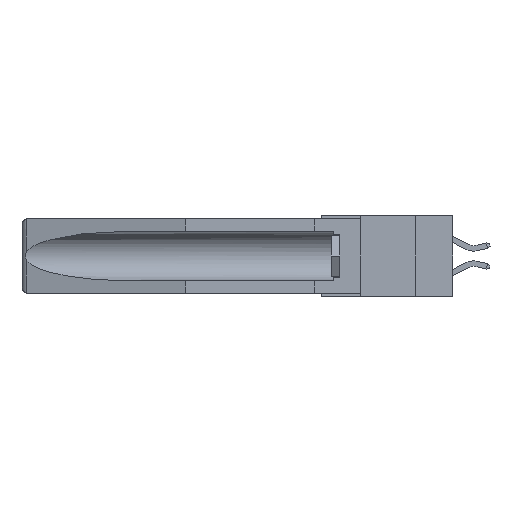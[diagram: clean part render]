
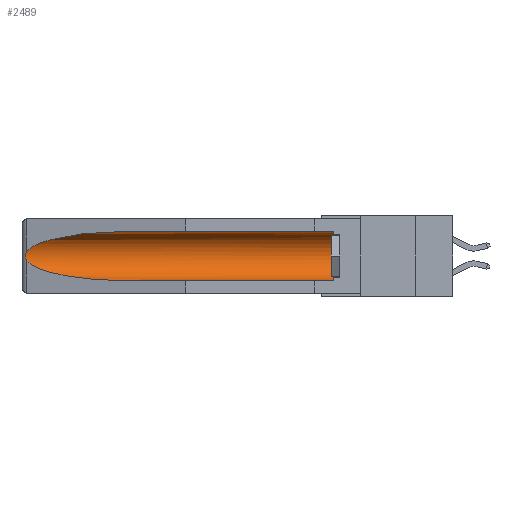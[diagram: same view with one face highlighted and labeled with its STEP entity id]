
A CAD part, left-side view. The second image highlights one B-rep face of the part: STEP entity #2489.
In plain terms, the highlighted cylindrical face has radius 2.857 mm (diameter 5.715 mm), a partial arc.
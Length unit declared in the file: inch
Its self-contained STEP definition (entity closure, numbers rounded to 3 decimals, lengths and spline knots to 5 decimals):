
#273 = VERTEX_POINT ( 'NONE', #5281 ) ;
#656 = EDGE_CURVE ( 'NONE', #273, #11229, #10351, .T. ) ;
#700 = LINE ( 'NONE', #4489, #19668 ) ;
#905 = CARTESIAN_POINT ( 'NONE',  ( 0.26537, 1.52718, -0.19328 ) ) ;
#1743 = EDGE_CURVE ( 'NONE', #6152, #273, #700, .T. ) ;
#2489 = ADVANCED_FACE ( 'NONE', ( #12251 ), #11237, .F. ) ;
#3765 = CARTESIAN_POINT ( 'NONE',  ( 0.26537, 1.52718, -0.19328 ) ) ;
#3939 = EDGE_CURVE ( 'NONE', #9594, #15477, #4488, .T. ) ;
#4488 =( BOUNDED_CURVE ( )  B_SPLINE_CURVE ( 3, ( #6036, #9517, #6104, #21020 ),
 .UNSPECIFIED., .F., .F. ) 
 B_SPLINE_CURVE_WITH_KNOTS ( ( 4, 4 ),
 ( 0.1948, 1.5708 ),
 .UNSPECIFIED. ) 
 CURVE ( )  GEOMETRIC_REPRESENTATION_ITEM ( )  RATIONAL_B_SPLINE_CURVE ( ( 1., 0.848, 0.848, 1. ) ) 
 REPRESENTATION_ITEM ( '' )  );
#4489 = CARTESIAN_POINT ( 'NONE',  ( 0.155, -0.30754, -0.059 ) ) ;
#5281 = CARTESIAN_POINT ( 'NONE',  ( 0.155, 1.07973, -0.059 ) ) ;
#5367 = CARTESIAN_POINT ( 'NONE',  ( 0.26537, 1.52718, -0.14972 ) ) ;
#5436 = LINE ( 'NONE', #8721, #10570 ) ;
#5533 = CARTESIAN_POINT ( 'NONE',  ( 0.2675, 1.53308, -0.16763 ) ) ;
#6036 = CARTESIAN_POINT ( 'NONE',  ( 0.26537, 1.52718, -0.19328 ) ) ;
#6104 = CARTESIAN_POINT ( 'NONE',  ( 0.21114, 1.30732, -0.284 ) ) ;
#6152 = VERTEX_POINT ( 'NONE', #14573 ) ;
#6284 = CIRCLE ( 'NONE', #19331, 0.1125 ) ;
#6410 = DIRECTION ( 'NONE',  ( 0., 0., 1. ) ) ;
#7042 = CARTESIAN_POINT ( 'NONE',  ( 0.2675, 1.53308, -0.17534 ) ) ;
#7171 = CARTESIAN_POINT ( 'NONE',  ( 0.26597, 1.5296, -0.19026 ) ) ;
#7842 = CARTESIAN_POINT ( 'NONE',  ( 0.155, 0.126, -0.1715 ) ) ;
#8088 = EDGE_CURVE ( 'NONE', #10126, #15477, #5436, .T. ) ;
#8093 = EDGE_CURVE ( 'NONE', #11229, #9594, #11219, .T. ) ;
#8721 = CARTESIAN_POINT ( 'NONE',  ( 0.155, -0.30754, -0.284 ) ) ;
#8939 = CARTESIAN_POINT ( 'NONE',  ( 0.2673, 1.53269, -0.17917 ) ) ;
#9015 = CARTESIAN_POINT ( 'NONE',  ( 0.26537, 1.52718, -0.14972 ) ) ;
#9180 = ORIENTED_EDGE ( 'NONE', *, *, #656, .T. ) ;
#9517 = CARTESIAN_POINT ( 'NONE',  ( 0.25451, 1.48313, -0.24835 ) ) ;
#9545 = CARTESIAN_POINT ( 'NONE',  ( 0.25451, 1.48313, -0.09465 ) ) ;
#9579 = DIRECTION ( 'NONE',  ( 0., 0., 1. ) ) ;
#9594 = VERTEX_POINT ( 'NONE', #905 ) ;
#9934 = ORIENTED_EDGE ( 'NONE', *, *, #1743, .T. ) ;
#10126 = VERTEX_POINT ( 'NONE', #10420 ) ;
#10351 =( BOUNDED_CURVE ( )  B_SPLINE_CURVE ( 3, ( #20422, #15564, #9545, #19484 ),
 .UNSPECIFIED., .F., .F. ) 
 B_SPLINE_CURVE_WITH_KNOTS ( ( 4, 4 ),
 ( 4.71239, 6.08839 ),
 .UNSPECIFIED. ) 
 CURVE ( )  GEOMETRIC_REPRESENTATION_ITEM ( )  RATIONAL_B_SPLINE_CURVE ( ( 1., 0.848, 0.848, 1. ) ) 
 REPRESENTATION_ITEM ( '' )  );
#10416 = CARTESIAN_POINT ( 'NONE',  ( 0.26654, 1.53092, -0.15636 ) ) ;
#10420 = CARTESIAN_POINT ( 'NONE',  ( 0.155, 0.126, -0.284 ) ) ;
#10570 = VECTOR ( 'NONE', #11985, 39.37008 ) ;
#10730 = AXIS2_PLACEMENT_3D ( 'NONE', #11189, #12803, #9579 ) ;
#10863 = ORIENTED_EDGE ( 'NONE', *, *, #3939, .T. ) ;
#11189 = CARTESIAN_POINT ( 'NONE',  ( 0.155, -0.30754, -0.1715 ) ) ;
#11219 = B_SPLINE_CURVE_WITH_KNOTS ( 'NONE', 3,
 ( #5367, #13760, #10416, #18748, #5533, #7042, #8939, #16961, #7171, #3765 ),
 .UNSPECIFIED., .F., .F.,
 ( 4, 2, 2, 2, 4 ),
 ( 0., 0.00029, 0.00058, 0.00087, 0.00117 ),
 .UNSPECIFIED. ) ;
#11220 = DIRECTION ( 'NONE',  ( 0., -1., 0. ) ) ;
#11229 = VERTEX_POINT ( 'NONE', #9015 ) ;
#11237 = CYLINDRICAL_SURFACE ( 'NONE', #10730, 0.1125 ) ;
#11288 = ORIENTED_EDGE ( 'NONE', *, *, #8093, .T. ) ;
#11985 = DIRECTION ( 'NONE',  ( 0., 1., 0. ) ) ;
#12251 = FACE_OUTER_BOUND ( 'NONE', #12893, .T. ) ;
#12384 = EDGE_CURVE ( 'NONE', #10126, #6152, #6284, .T. ) ;
#12796 = CARTESIAN_POINT ( 'NONE',  ( 0.155, 1.07973, -0.284 ) ) ;
#12803 = DIRECTION ( 'NONE',  ( 0., 1., 0. ) ) ;
#12893 = EDGE_LOOP ( 'NONE', ( #9180, #11288, #10863, #15803, #14652, #9934 ) ) ;
#13760 = CARTESIAN_POINT ( 'NONE',  ( 0.26597, 1.52961, -0.15275 ) ) ;
#14573 = CARTESIAN_POINT ( 'NONE',  ( 0.155, 0.126, -0.059 ) ) ;
#14652 = ORIENTED_EDGE ( 'NONE', *, *, #12384, .T. ) ;
#15477 = VERTEX_POINT ( 'NONE', #12796 ) ;
#15564 = CARTESIAN_POINT ( 'NONE',  ( 0.21114, 1.30732, -0.059 ) ) ;
#15803 = ORIENTED_EDGE ( 'NONE', *, *, #8088, .F. ) ;
#16961 = CARTESIAN_POINT ( 'NONE',  ( 0.26655, 1.53094, -0.18657 ) ) ;
#18748 = CARTESIAN_POINT ( 'NONE',  ( 0.2673, 1.5327, -0.16383 ) ) ;
#19331 = AXIS2_PLACEMENT_3D ( 'NONE', #7842, #11220, #6410 ) ;
#19484 = CARTESIAN_POINT ( 'NONE',  ( 0.26537, 1.52718, -0.14972 ) ) ;
#19668 = VECTOR ( 'NONE', #20958, 39.37008 ) ;
#20422 = CARTESIAN_POINT ( 'NONE',  ( 0.155, 1.07973, -0.059 ) ) ;
#20958 = DIRECTION ( 'NONE',  ( 0., 1., 0. ) ) ;
#21020 = CARTESIAN_POINT ( 'NONE',  ( 0.155, 1.07973, -0.284 ) ) ;
